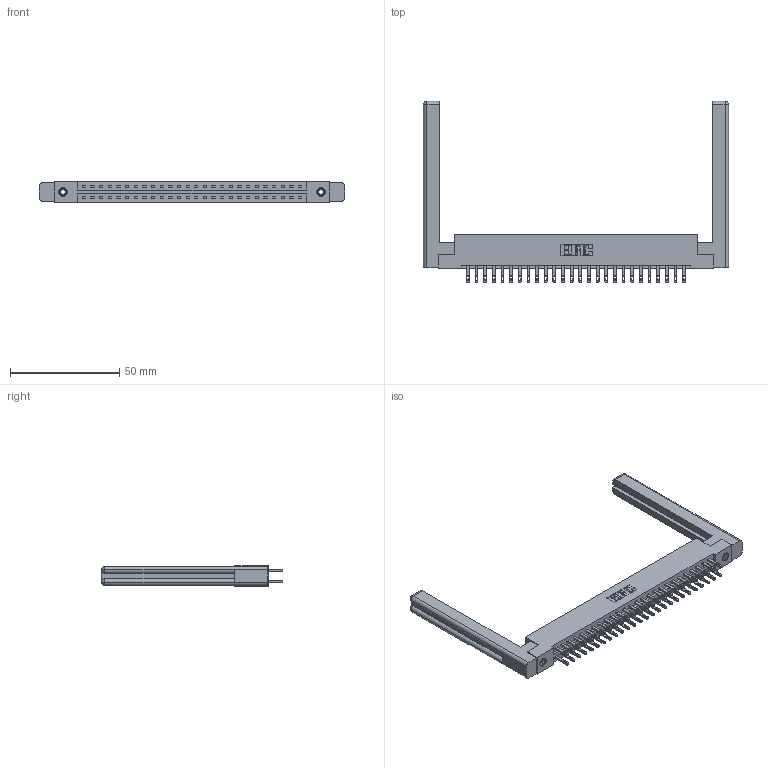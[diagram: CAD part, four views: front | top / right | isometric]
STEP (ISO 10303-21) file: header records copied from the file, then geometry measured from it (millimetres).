
FILE_DESCRIPTION (( 'STEP AP203' ), '1' );
FILE_NAME ('337-052-500-258.STEP', '2019-10-09T16:28:31', ( '' ), ( '' ), 'SwSTEP 2.0', 'SolidWorks 2016', '' );
FILE_SCHEMA (( 'CONFIG_CONTROL_DESIGN' ));
Length unit declared in the file: inch
Products named in the file (5): 307-220-058; 337 Part_Flush Mounting Lugs - 0.156 Dia-TI; 345-292-001_345-293-100; 337-052-500-258; 345-250-001_345-250-001-102
Assembly tree (57 placements, depth 2):
  337-052-500-258
    337 Part_Flush Mounting Lugs - 0.156 Dia-TI
    345-292-001_345-293-100  x52
    345-250-001_345-250-001-102  x2
    307-220-058  x2
Bounding box: 139.65 x 82.94 x 9.4 mm (x, y, z)
Volume: 21805.6 mm3; surface area: 22045.2 mm2
Topology: 57 solids, 57 shells, 2856 faces, 8621 edges, 5734 vertices
Faces by surface type: plane 1818, cylinder 1014, cone 12, torus 12
Entity records: 24792 total; most frequent: CARTESIAN_POINT 4197, ORIENTED_EDGE 4072, DIRECTION 3616, EDGE_CURVE 2036, VECTOR 1856, LINE 1856, VERTEX_POINT 1350, AXIS2_PLACEMENT_3D 880
